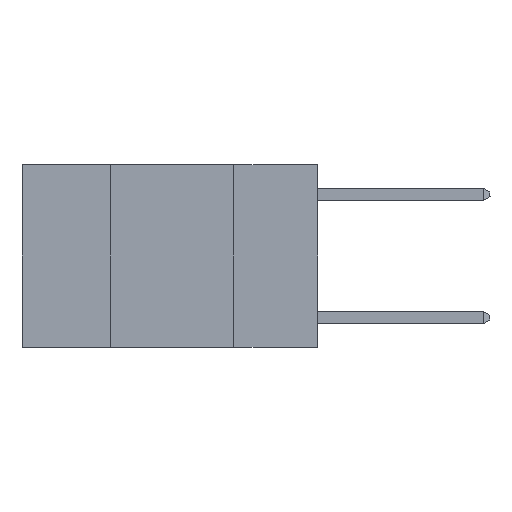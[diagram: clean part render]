
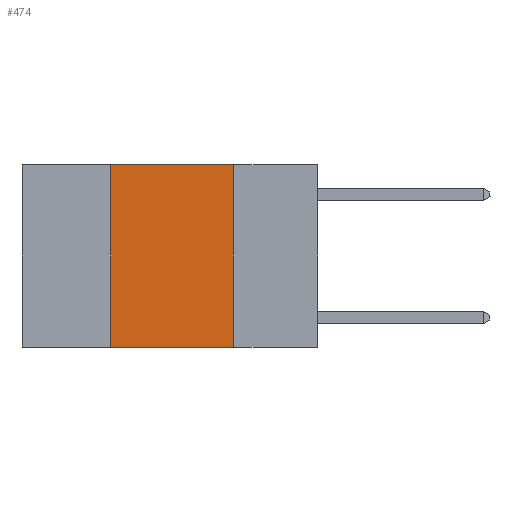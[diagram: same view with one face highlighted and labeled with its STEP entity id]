
A CAD part, left-side view. The second image highlights one B-rep face of the part: STEP entity #474.
In plain terms, the highlighted planar face has unit normal (-1, 0, 0).
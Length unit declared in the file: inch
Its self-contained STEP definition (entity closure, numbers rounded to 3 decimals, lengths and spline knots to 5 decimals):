
#474 = ADVANCED_FACE ( 'NONE', ( #14768 ), #14512, .F. ) ;
#614 = VERTEX_POINT ( 'NONE', #9412 ) ;
#729 = VERTEX_POINT ( 'NONE', #3648 ) ;
#817 = CARTESIAN_POINT ( 'NONE',  ( 0., 0.6, 0. ) ) ;
#905 = DIRECTION ( 'NONE',  ( 0., 0., 1. ) ) ;
#1063 = EDGE_CURVE ( 'NONE', #2344, #729, #9618, .T. ) ;
#2289 = DIRECTION ( 'NONE',  ( 0., -1., 0. ) ) ;
#2325 = ORIENTED_EDGE ( 'NONE', *, *, #13853, .F. ) ;
#2344 = VERTEX_POINT ( 'NONE', #4429 ) ;
#2374 = EDGE_CURVE ( 'NONE', #15301, #729, #12900, .T. ) ;
#3648 = CARTESIAN_POINT ( 'NONE',  ( 0., 0.17, -0.37 ) ) ;
#4394 = VECTOR ( 'NONE', #2289, 39.37008 ) ;
#4401 = DIRECTION ( 'NONE',  ( 0., 0., -1. ) ) ;
#4429 = CARTESIAN_POINT ( 'NONE',  ( 0., 0.17, 0. ) ) ;
#4621 = CARTESIAN_POINT ( 'NONE',  ( 0., 0.17, 0. ) ) ;
#5457 = ORIENTED_EDGE ( 'NONE', *, *, #14198, .F. ) ;
#5644 = AXIS2_PLACEMENT_3D ( 'NONE', #6960, #9044, #15094 ) ;
#6960 = CARTESIAN_POINT ( 'NONE',  ( 0., 0.6, 0. ) ) ;
#7566 = CARTESIAN_POINT ( 'NONE',  ( 0., 0.42, 0. ) ) ;
#8743 = VECTOR ( 'NONE', #905, 39.37008 ) ;
#9044 = DIRECTION ( 'NONE',  ( 1., 0., 0. ) ) ;
#9230 = VECTOR ( 'NONE', #4401, 39.37008 ) ;
#9247 = ORIENTED_EDGE ( 'NONE', *, *, #2374, .T. ) ;
#9412 = CARTESIAN_POINT ( 'NONE',  ( 0., 0.42, 0. ) ) ;
#9618 = LINE ( 'NONE', #4621, #9230 ) ;
#10608 = ORIENTED_EDGE ( 'NONE', *, *, #1063, .F. ) ;
#10822 = CARTESIAN_POINT ( 'NONE',  ( 0., 0.6, -0.37 ) ) ;
#12057 = DIRECTION ( 'NONE',  ( 0., -1., 0. ) ) ;
#12067 = LINE ( 'NONE', #7566, #8743 ) ;
#12900 = LINE ( 'NONE', #10822, #16697 ) ;
#13471 = CARTESIAN_POINT ( 'NONE',  ( 0., 0.42, -0.37 ) ) ;
#13853 = EDGE_CURVE ( 'NONE', #15301, #614, #12067, .T. ) ;
#14198 = EDGE_CURVE ( 'NONE', #614, #2344, #14451, .T. ) ;
#14451 = LINE ( 'NONE', #817, #4394 ) ;
#14512 = PLANE ( 'NONE',  #5644 ) ;
#14768 = FACE_OUTER_BOUND ( 'NONE', #16217, .T. ) ;
#15094 = DIRECTION ( 'NONE',  ( 0., 0., -1. ) ) ;
#15301 = VERTEX_POINT ( 'NONE', #13471 ) ;
#16217 = EDGE_LOOP ( 'NONE', ( #10608, #5457, #2325, #9247 ) ) ;
#16697 = VECTOR ( 'NONE', #12057, 39.37008 ) ;
